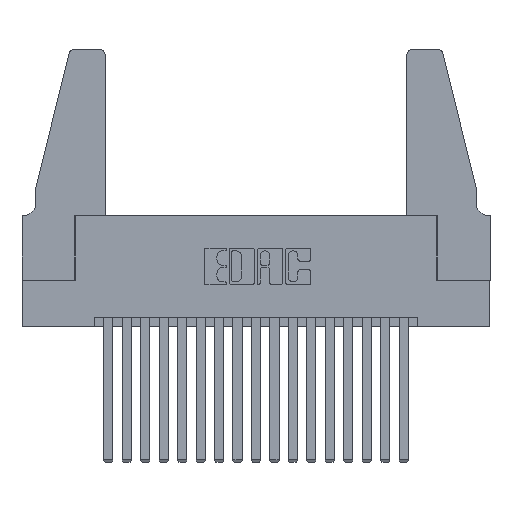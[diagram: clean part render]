
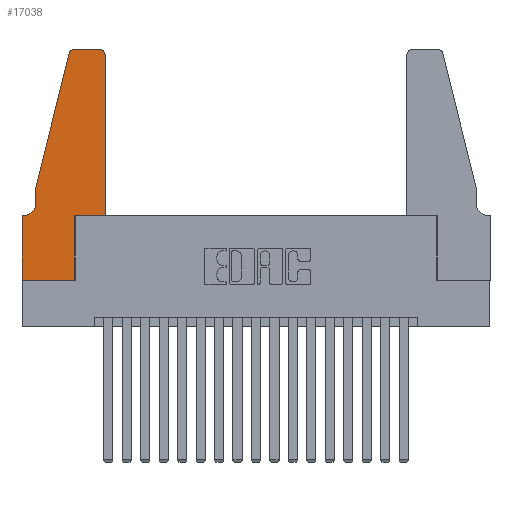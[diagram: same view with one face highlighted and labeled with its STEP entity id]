
A CAD part, top view. The second image highlights one B-rep face of the part: STEP entity #17038.
In plain terms, the highlighted planar face has unit normal (0, 0, 1).
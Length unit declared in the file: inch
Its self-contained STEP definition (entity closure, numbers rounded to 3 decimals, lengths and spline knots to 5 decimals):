
#8 = VECTOR ( 'NONE', #16242, 39.37008 ) ;
#36 = CARTESIAN_POINT ( 'NONE',  ( 0.4205, 1.25, 0.37 ) ) ;
#219 = ORIENTED_EDGE ( 'NONE', *, *, #13140, .T. ) ;
#913 = CARTESIAN_POINT ( 'NONE',  ( 0.0055, 0.35, 0.37 ) ) ;
#1044 = LINE ( 'NONE', #2754, #15951 ) ;
#1077 = CARTESIAN_POINT ( 'NONE',  ( 0.2605, 1.25, 0.37 ) ) ;
#1377 = ORIENTED_EDGE ( 'NONE', *, *, #16674, .T. ) ;
#1611 = CIRCLE ( 'NONE', #4398, 0.03 ) ;
#1807 = CARTESIAN_POINT ( 'NONE',  ( 0., 0., 0.37 ) ) ;
#2066 = VERTEX_POINT ( 'NONE', #3455 ) ;
#2315 = EDGE_CURVE ( 'NONE', #8388, #6796, #13492, .T. ) ;
#2754 = CARTESIAN_POINT ( 'NONE',  ( 0.0755, 0.35, 0.37 ) ) ;
#2866 = CARTESIAN_POINT ( 'NONE',  ( 0., 0.35, 0.37 ) ) ;
#3455 = CARTESIAN_POINT ( 'NONE',  ( 0., 0.35, 0.37 ) ) ;
#3528 = ORIENTED_EDGE ( 'NONE', *, *, #7248, .T. ) ;
#3784 = CARTESIAN_POINT ( 'NONE',  ( 0.2865, 0., 0.37 ) ) ;
#3835 = EDGE_CURVE ( 'NONE', #14578, #15751, #3924, .T. ) ;
#3924 = LINE ( 'NONE', #1807, #8 ) ;
#3939 = DIRECTION ( 'NONE',  ( -1., 0., 0. ) ) ;
#4047 = ORIENTED_EDGE ( 'NONE', *, *, #7768, .T. ) ;
#4267 = VERTEX_POINT ( 'NONE', #11488 ) ;
#4277 = DIRECTION ( 'NONE',  ( 0., 0., 1. ) ) ;
#4325 = CARTESIAN_POINT ( 'NONE',  ( 0., 0., 0.37 ) ) ;
#4328 = DIRECTION ( 'NONE',  ( 1., 0., 0. ) ) ;
#4398 = AXIS2_PLACEMENT_3D ( 'NONE', #4728, #14805, #6173 ) ;
#4728 = CARTESIAN_POINT ( 'NONE',  ( 0.284, 1.22, 0.37 ) ) ;
#4792 = LINE ( 'NONE', #1077, #7693 ) ;
#5204 = EDGE_LOOP ( 'NONE', ( #16142, #16711, #7619, #1377, #16286, #9259, #219, #15935, #3528, #17170, #11776, #4047 ) ) ;
#5483 = DIRECTION ( 'NONE',  ( -0.239, -0.971, 0. ) ) ;
#5666 = EDGE_CURVE ( 'NONE', #8003, #4267, #14421, .T. ) ;
#5772 = EDGE_CURVE ( 'NONE', #15769, #2066, #1044, .T. ) ;
#5808 = VECTOR ( 'NONE', #18262, 39.37008 ) ;
#5843 = CARTESIAN_POINT ( 'NONE',  ( 0.284, 1.25, 0.37 ) ) ;
#5974 = CARTESIAN_POINT ( 'NONE',  ( 0.0055, 0.42, 0.37 ) ) ;
#6061 = DIRECTION ( 'NONE',  ( 0., 1., 0. ) ) ;
#6173 = DIRECTION ( 'NONE',  ( 1., 0., 0. ) ) ;
#6367 = LINE ( 'NONE', #16046, #13622 ) ;
#6715 = VECTOR ( 'NONE', #5483, 39.37008 ) ;
#6796 = VERTEX_POINT ( 'NONE', #16574 ) ;
#7145 = PLANE ( 'NONE',  #14116 ) ;
#7248 = EDGE_CURVE ( 'NONE', #15751, #8818, #17689, .T. ) ;
#7409 = DIRECTION ( 'NONE',  ( -1., 0., 0. ) ) ;
#7619 = ORIENTED_EDGE ( 'NONE', *, *, #5666, .T. ) ;
#7693 = VECTOR ( 'NONE', #3939, 39.37008 ) ;
#7768 = EDGE_CURVE ( 'NONE', #6796, #18441, #16789, .T. ) ;
#8003 = VERTEX_POINT ( 'NONE', #17945 ) ;
#8388 = VERTEX_POINT ( 'NONE', #16764 ) ;
#8818 = VERTEX_POINT ( 'NONE', #17670 ) ;
#9259 = ORIENTED_EDGE ( 'NONE', *, *, #5772, .T. ) ;
#9583 = VECTOR ( 'NONE', #13047, 39.37008 ) ;
#9631 = CARTESIAN_POINT ( 'NONE',  ( 0., 0., 0.37 ) ) ;
#9963 = EDGE_CURVE ( 'NONE', #17578, #15769, #16704, .T. ) ;
#11378 = AXIS2_PLACEMENT_3D ( 'NONE', #5974, #16039, #7409 ) ;
#11488 = CARTESIAN_POINT ( 'NONE',  ( 0.0755, 0.5, 0.37 ) ) ;
#11776 = ORIENTED_EDGE ( 'NONE', *, *, #2315, .T. ) ;
#11974 = AXIS2_PLACEMENT_3D ( 'NONE', #12943, #4277, #14382 ) ;
#12943 = CARTESIAN_POINT ( 'NONE',  ( 0.4205, 1.22, 0.37 ) ) ;
#12992 = DIRECTION ( 'NONE',  ( 0., 0., 1. ) ) ;
#13047 = DIRECTION ( 'NONE',  ( 0., -1., 0. ) ) ;
#13140 = EDGE_CURVE ( 'NONE', #2066, #14578, #13435, .T. ) ;
#13148 = VERTEX_POINT ( 'NONE', #5843 ) ;
#13271 = CARTESIAN_POINT ( 'NONE',  ( 0.2865, 0.35, 0.37 ) ) ;
#13297 = VECTOR ( 'NONE', #17248, 39.37008 ) ;
#13435 = LINE ( 'NONE', #4325, #9583 ) ;
#13492 = LINE ( 'NONE', #16898, #5808 ) ;
#13622 = VECTOR ( 'NONE', #16108, 39.37008 ) ;
#13749 = LINE ( 'NONE', #15835, #13297 ) ;
#14084 = FACE_OUTER_BOUND ( 'NONE', #5204, .T. ) ;
#14116 = AXIS2_PLACEMENT_3D ( 'NONE', #2866, #12992, #4328 ) ;
#14149 = CARTESIAN_POINT ( 'NONE',  ( 0.0755, 0.5, 0.37 ) ) ;
#14253 = EDGE_CURVE ( 'NONE', #8818, #8388, #6367, .T. ) ;
#14304 = EDGE_CURVE ( 'NONE', #13148, #8003, #1611, .T. ) ;
#14382 = DIRECTION ( 'NONE',  ( 1., 0., 0. ) ) ;
#14421 = LINE ( 'NONE', #14149, #6715 ) ;
#14578 = VERTEX_POINT ( 'NONE', #9631 ) ;
#14635 = EDGE_CURVE ( 'NONE', #18441, #13148, #4792, .T. ) ;
#14805 = DIRECTION ( 'NONE',  ( 0., 0., 1. ) ) ;
#14822 = VECTOR ( 'NONE', #6061, 39.37008 ) ;
#15445 = CARTESIAN_POINT ( 'NONE',  ( 0.0755, 0.42, 0.37 ) ) ;
#15751 = VERTEX_POINT ( 'NONE', #3784 ) ;
#15769 = VERTEX_POINT ( 'NONE', #913 ) ;
#15835 = CARTESIAN_POINT ( 'NONE',  ( 0.0755, 0.5, 0.37 ) ) ;
#15935 = ORIENTED_EDGE ( 'NONE', *, *, #3835, .T. ) ;
#15951 = VECTOR ( 'NONE', #18581, 39.37008 ) ;
#16039 = DIRECTION ( 'NONE',  ( 0., 0., -1. ) ) ;
#16046 = CARTESIAN_POINT ( 'NONE',  ( 0.4505, 0.35, 0.37 ) ) ;
#16108 = DIRECTION ( 'NONE',  ( 1., 0., 0. ) ) ;
#16142 = ORIENTED_EDGE ( 'NONE', *, *, #14635, .T. ) ;
#16242 = DIRECTION ( 'NONE',  ( 1., 0., 0. ) ) ;
#16286 = ORIENTED_EDGE ( 'NONE', *, *, #9963, .T. ) ;
#16574 = CARTESIAN_POINT ( 'NONE',  ( 0.4505, 1.22, 0.37 ) ) ;
#16674 = EDGE_CURVE ( 'NONE', #4267, #17578, #13749, .T. ) ;
#16704 = CIRCLE ( 'NONE', #11378, 0.07 ) ;
#16711 = ORIENTED_EDGE ( 'NONE', *, *, #14304, .T. ) ;
#16764 = CARTESIAN_POINT ( 'NONE',  ( 0.4505, 0.35, 0.37 ) ) ;
#16789 = CIRCLE ( 'NONE', #11974, 0.03 ) ;
#16898 = CARTESIAN_POINT ( 'NONE',  ( 0.4505, 0.35, 0.37 ) ) ;
#17038 = ADVANCED_FACE ( 'NONE', ( #14084 ), #7145, .T. ) ;
#17170 = ORIENTED_EDGE ( 'NONE', *, *, #14253, .T. ) ;
#17248 = DIRECTION ( 'NONE',  ( 0., -1., 0. ) ) ;
#17578 = VERTEX_POINT ( 'NONE', #15445 ) ;
#17670 = CARTESIAN_POINT ( 'NONE',  ( 0.2865, 0.35, 0.37 ) ) ;
#17689 = LINE ( 'NONE', #13271, #14822 ) ;
#17945 = CARTESIAN_POINT ( 'NONE',  ( 0.25487, 1.22718, 0.37 ) ) ;
#18262 = DIRECTION ( 'NONE',  ( 0., 1., 0. ) ) ;
#18441 = VERTEX_POINT ( 'NONE', #36 ) ;
#18581 = DIRECTION ( 'NONE',  ( -1., 0., 0. ) ) ;
